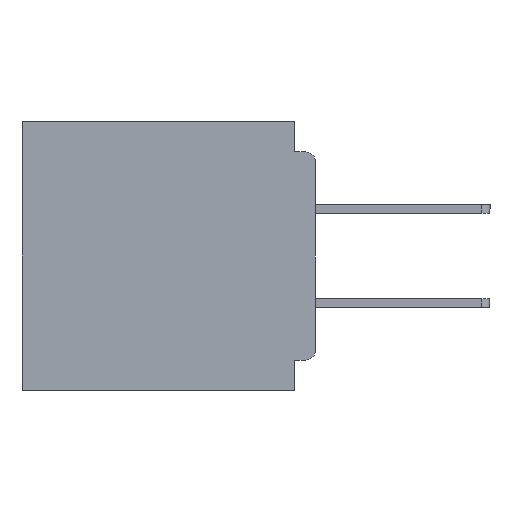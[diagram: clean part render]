
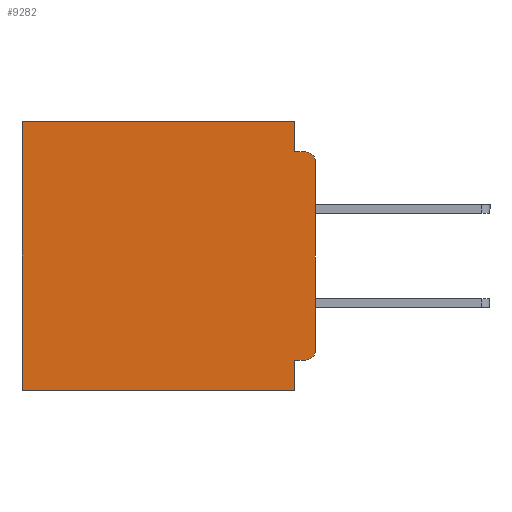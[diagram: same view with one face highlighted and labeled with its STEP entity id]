
A CAD part, left-side view. The second image highlights one B-rep face of the part: STEP entity #9282.
In plain terms, the highlighted planar face has unit normal (-1, 0, 0).
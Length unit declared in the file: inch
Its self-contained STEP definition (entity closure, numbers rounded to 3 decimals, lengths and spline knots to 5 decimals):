
#84 = DIRECTION ( 'NONE',  ( 0., 0., -1. ) ) ;
#1692 = EDGE_LOOP ( 'NONE', ( #18918, #46911, #41404, #34408, #24822, #12821, #18681, #29515, #46836, #10156 ) ) ;
#2310 = VECTOR ( 'NONE', #32061, 39.37008 ) ;
#2854 = VECTOR ( 'NONE', #38445, 39.37008 ) ;
#3413 = VECTOR ( 'NONE', #17615, 39.37008 ) ;
#5149 = DIRECTION ( 'NONE',  ( -1., 0., 0. ) ) ;
#5364 = VERTEX_POINT ( 'NONE', #33523 ) ;
#5710 = EDGE_CURVE ( 'NONE', #45472, #28283, #34379, .T. ) ;
#6473 = CARTESIAN_POINT ( 'NONE',  ( 0.3, 0., -0.34 ) ) ;
#6767 = CARTESIAN_POINT ( 'NONE',  ( 0.3, 0.437, -0.4 ) ) ;
#6883 = CARTESIAN_POINT ( 'NONE',  ( 0.3, 0., -0.4 ) ) ;
#7063 = VECTOR ( 'NONE', #33905, 39.37008 ) ;
#7085 = VECTOR ( 'NONE', #39482, 39.37008 ) ;
#7858 = VERTEX_POINT ( 'NONE', #6473 ) ;
#8792 = EDGE_CURVE ( 'NONE', #5364, #41137, #27455, .T. ) ;
#8935 = CARTESIAN_POINT ( 'NONE',  ( 0.3, 0., 0. ) ) ;
#9282 = ADVANCED_FACE ( 'NONE', ( #32799 ), #44869, .F. ) ;
#9779 = VECTOR ( 'NONE', #38536, 39.37008 ) ;
#10156 = ORIENTED_EDGE ( 'NONE', *, *, #30593, .T. ) ;
#10755 = DIRECTION ( 'NONE',  ( 0., 0., -1. ) ) ;
#10957 = CARTESIAN_POINT ( 'NONE',  ( 0.3, 0.031, -0.4 ) ) ;
#11221 = LINE ( 'NONE', #31981, #20196 ) ;
#11638 = EDGE_CURVE ( 'NONE', #45472, #7858, #23841, .T. ) ;
#12142 = EDGE_CURVE ( 'NONE', #32205, #5364, #11221, .T. ) ;
#12192 = LINE ( 'NONE', #15660, #9779 ) ;
#12527 = CARTESIAN_POINT ( 'NONE',  ( 0.3, 0.031, -0.045 ) ) ;
#12821 = ORIENTED_EDGE ( 'NONE', *, *, #32098, .T. ) ;
#12876 = DIRECTION ( 'NONE',  ( 0., 1., 0. ) ) ;
#13098 = LINE ( 'NONE', #19426, #2854 ) ;
#13445 = CARTESIAN_POINT ( 'NONE',  ( 0.3, 0.015, -0.355 ) ) ;
#13673 = DIRECTION ( 'NONE',  ( 0., 1., 0. ) ) ;
#14456 = CIRCLE ( 'NONE', #35215, 0.015 ) ;
#15660 = CARTESIAN_POINT ( 'NONE',  ( 0.3, 0.031, 0. ) ) ;
#15703 = VERTEX_POINT ( 'NONE', #6767 ) ;
#17095 = CARTESIAN_POINT ( 'NONE',  ( 0.3, 0.031, 0. ) ) ;
#17453 = CARTESIAN_POINT ( 'NONE',  ( 0.3, 0., -0.4 ) ) ;
#17615 = DIRECTION ( 'NONE',  ( 0., 0., -1. ) ) ;
#17656 = EDGE_CURVE ( 'NONE', #27442, #28334, #22740, .T. ) ;
#18681 = ORIENTED_EDGE ( 'NONE', *, *, #33528, .F. ) ;
#18918 = ORIENTED_EDGE ( 'NONE', *, *, #11638, .F. ) ;
#19426 = CARTESIAN_POINT ( 'NONE',  ( 0.3, 0., -0.045 ) ) ;
#20196 = VECTOR ( 'NONE', #12876, 39.37008 ) ;
#22740 = LINE ( 'NONE', #8935, #2310 ) ;
#23089 = DIRECTION ( 'NONE',  ( -1., 0., 0. ) ) ;
#23841 = LINE ( 'NONE', #17453, #3413 ) ;
#24542 = VERTEX_POINT ( 'NONE', #12527 ) ;
#24822 = ORIENTED_EDGE ( 'NONE', *, *, #17656, .T. ) ;
#27442 = VERTEX_POINT ( 'NONE', #17095 ) ;
#27455 = LINE ( 'NONE', #10957, #7063 ) ;
#27479 = LINE ( 'NONE', #31752, #7085 ) ;
#28123 = CARTESIAN_POINT ( 'NONE',  ( 0.3, 0.015, -0.06 ) ) ;
#28283 = VERTEX_POINT ( 'NONE', #48758 ) ;
#28334 = VERTEX_POINT ( 'NONE', #45275 ) ;
#29342 = EDGE_CURVE ( 'NONE', #27442, #24542, #12192, .T. ) ;
#29515 = ORIENTED_EDGE ( 'NONE', *, *, #8792, .F. ) ;
#30593 = EDGE_CURVE ( 'NONE', #32205, #7858, #14456, .T. ) ;
#31548 = LINE ( 'NONE', #44777, #41565 ) ;
#31752 = CARTESIAN_POINT ( 'NONE',  ( 0.3, 0.437, -0.4 ) ) ;
#31979 = DIRECTION ( 'NONE',  ( 0., 0., -1. ) ) ;
#31981 = CARTESIAN_POINT ( 'NONE',  ( 0.3, 0., -0.355 ) ) ;
#32061 = DIRECTION ( 'NONE',  ( 0., 1., 0. ) ) ;
#32098 = EDGE_CURVE ( 'NONE', #28334, #15703, #27479, .T. ) ;
#32205 = VERTEX_POINT ( 'NONE', #13445 ) ;
#32799 = FACE_OUTER_BOUND ( 'NONE', #1692, .T. ) ;
#33087 = CARTESIAN_POINT ( 'NONE',  ( 0.3, 0.031, -0.4 ) ) ;
#33523 = CARTESIAN_POINT ( 'NONE',  ( 0.3, 0.031, -0.355 ) ) ;
#33528 = EDGE_CURVE ( 'NONE', #41137, #15703, #31548, .T. ) ;
#33715 = DIRECTION ( 'NONE',  ( 1., 0., 0. ) ) ;
#33905 = DIRECTION ( 'NONE',  ( 0., 0., -1. ) ) ;
#34379 = CIRCLE ( 'NONE', #48939, 0.015 ) ;
#34408 = ORIENTED_EDGE ( 'NONE', *, *, #29342, .F. ) ;
#35215 = AXIS2_PLACEMENT_3D ( 'NONE', #45826, #23089, #84 ) ;
#37180 = EDGE_CURVE ( 'NONE', #24542, #28283, #13098, .T. ) ;
#38445 = DIRECTION ( 'NONE',  ( 0., -1., 0. ) ) ;
#38536 = DIRECTION ( 'NONE',  ( 0., 0., -1. ) ) ;
#39482 = DIRECTION ( 'NONE',  ( 0., 0., -1. ) ) ;
#41137 = VERTEX_POINT ( 'NONE', #33087 ) ;
#41404 = ORIENTED_EDGE ( 'NONE', *, *, #37180, .F. ) ;
#41565 = VECTOR ( 'NONE', #13673, 39.37008 ) ;
#43384 = CARTESIAN_POINT ( 'NONE',  ( 0.3, 0., -0.06 ) ) ;
#44777 = CARTESIAN_POINT ( 'NONE',  ( 0.3, 0., -0.4 ) ) ;
#44869 = PLANE ( 'NONE',  #47749 ) ;
#45275 = CARTESIAN_POINT ( 'NONE',  ( 0.3, 0.437, 0. ) ) ;
#45472 = VERTEX_POINT ( 'NONE', #43384 ) ;
#45826 = CARTESIAN_POINT ( 'NONE',  ( 0.3, 0.015, -0.34 ) ) ;
#46836 = ORIENTED_EDGE ( 'NONE', *, *, #12142, .F. ) ;
#46911 = ORIENTED_EDGE ( 'NONE', *, *, #5710, .T. ) ;
#47749 = AXIS2_PLACEMENT_3D ( 'NONE', #6883, #33715, #10755 ) ;
#48758 = CARTESIAN_POINT ( 'NONE',  ( 0.3, 0.015, -0.045 ) ) ;
#48939 = AXIS2_PLACEMENT_3D ( 'NONE', #28123, #5149, #31979 ) ;
